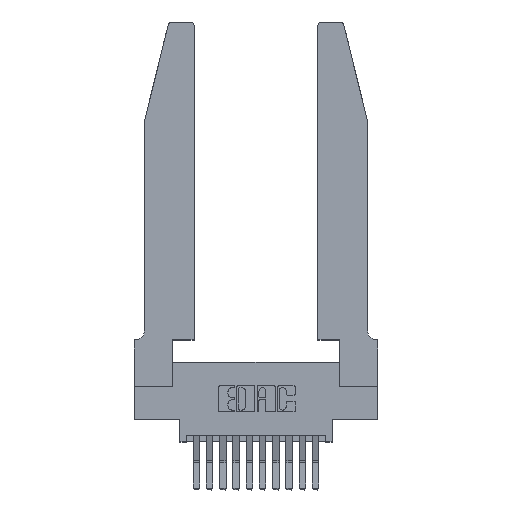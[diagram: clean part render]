
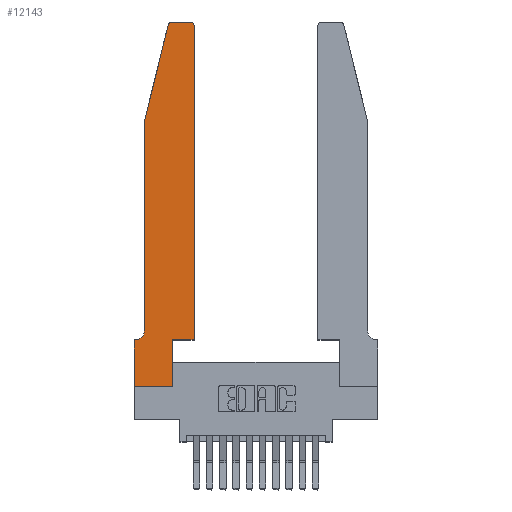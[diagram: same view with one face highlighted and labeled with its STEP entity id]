
A CAD part, top view. The second image highlights one B-rep face of the part: STEP entity #12143.
In plain terms, the highlighted planar face has unit normal (0, 0, 1).
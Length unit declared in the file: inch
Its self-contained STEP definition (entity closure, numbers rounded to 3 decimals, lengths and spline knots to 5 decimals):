
#3 = VERTEX_POINT ( 'NONE', #9684 ) ;
#420 = LINE ( 'NONE', #16414, #14131 ) ;
#710 = ORIENTED_EDGE ( 'NONE', *, *, #14507, .T. ) ;
#722 = DIRECTION ( 'NONE',  ( 1., 0., 0. ) ) ;
#805 = VERTEX_POINT ( 'NONE', #4292 ) ;
#1118 = DIRECTION ( 'NONE',  ( -1., 0., 0. ) ) ;
#1299 = EDGE_CURVE ( 'NONE', #12303, #10691, #420, .T. ) ;
#1308 = CARTESIAN_POINT ( 'NONE',  ( 0.4505, 0.35, 0.37 ) ) ;
#1601 = ORIENTED_EDGE ( 'NONE', *, *, #2215, .T. ) ;
#2215 = EDGE_CURVE ( 'NONE', #4727, #5094, #15937, .T. ) ;
#2238 = CARTESIAN_POINT ( 'NONE',  ( 0.0755, 2., 0.37 ) ) ;
#2670 = CARTESIAN_POINT ( 'NONE',  ( 0.0055, 0.35, 0.37 ) ) ;
#2739 = LINE ( 'NONE', #3442, #13275 ) ;
#3157 = LINE ( 'NONE', #16989, #16668 ) ;
#3193 = VERTEX_POINT ( 'NONE', #8471 ) ;
#3205 = ORIENTED_EDGE ( 'NONE', *, *, #13004, .T. ) ;
#3220 = CARTESIAN_POINT ( 'NONE',  ( 0.0755, 2., 0.37 ) ) ;
#3237 = LINE ( 'NONE', #15330, #13325 ) ;
#3442 = CARTESIAN_POINT ( 'NONE',  ( 0., 0., 0.37 ) ) ;
#3462 = ORIENTED_EDGE ( 'NONE', *, *, #9784, .T. ) ;
#3712 = ORIENTED_EDGE ( 'NONE', *, *, #1299, .T. ) ;
#3926 = CARTESIAN_POINT ( 'NONE',  ( 0., 0., 0.37 ) ) ;
#4292 = CARTESIAN_POINT ( 'NONE',  ( 0.2865, 0., 0.37 ) ) ;
#4449 = ORIENTED_EDGE ( 'NONE', *, *, #14977, .T. ) ;
#4578 = EDGE_LOOP ( 'NONE', ( #3462, #12439, #3205, #4449, #11653, #3712, #5578, #15171, #8110, #15825, #710, #1601 ) ) ;
#4727 = VERTEX_POINT ( 'NONE', #11401 ) ;
#4792 = DIRECTION ( 'NONE',  ( -0.239, -0.971, 0. ) ) ;
#5094 = VERTEX_POINT ( 'NONE', #14942 ) ;
#5296 = DIRECTION ( 'NONE',  ( 1., 0., 0. ) ) ;
#5457 = AXIS2_PLACEMENT_3D ( 'NONE', #6131, #8782, #722 ) ;
#5578 = ORIENTED_EDGE ( 'NONE', *, *, #13606, .T. ) ;
#5979 = AXIS2_PLACEMENT_3D ( 'NONE', #15383, #7617, #16695 ) ;
#6131 = CARTESIAN_POINT ( 'NONE',  ( 0., 0.35, 0.37 ) ) ;
#6413 = DIRECTION ( 'NONE',  ( 0., 1., 0. ) ) ;
#6873 = CARTESIAN_POINT ( 'NONE',  ( 0.0755, 2., 0.37 ) ) ;
#7020 = EDGE_CURVE ( 'NONE', #9657, #12303, #12777, .T. ) ;
#7208 = DIRECTION ( 'NONE',  ( 0., 0., -1. ) ) ;
#7261 = EDGE_CURVE ( 'NONE', #14782, #3, #12577, .T. ) ;
#7352 = PLANE ( 'NONE',  #5457 ) ;
#7617 = DIRECTION ( 'NONE',  ( 0., 0., 1. ) ) ;
#8110 = ORIENTED_EDGE ( 'NONE', *, *, #15458, .T. ) ;
#8471 = CARTESIAN_POINT ( 'NONE',  ( 0., 0., 0.37 ) ) ;
#8506 = VERTEX_POINT ( 'NONE', #6873 ) ;
#8766 = CARTESIAN_POINT ( 'NONE',  ( 0.284, 2.75, 0.37 ) ) ;
#8782 = DIRECTION ( 'NONE',  ( 0., 0., 1. ) ) ;
#9070 = VECTOR ( 'NONE', #5296, 39.37008 ) ;
#9521 = LINE ( 'NONE', #3220, #16013 ) ;
#9524 = VERTEX_POINT ( 'NONE', #16996 ) ;
#9657 = VERTEX_POINT ( 'NONE', #12226 ) ;
#9684 = CARTESIAN_POINT ( 'NONE',  ( 0.4505, 0.35, 0.37 ) ) ;
#9725 = LINE ( 'NONE', #12959, #13215 ) ;
#9784 = EDGE_CURVE ( 'NONE', #5094, #10909, #3237, .T. ) ;
#9810 = EDGE_CURVE ( 'NONE', #10909, #9524, #9826, .T. ) ;
#9826 = CIRCLE ( 'NONE', #5979, 0.03 ) ;
#10176 = DIRECTION ( 'NONE',  ( 0., -1., 0. ) ) ;
#10691 = VERTEX_POINT ( 'NONE', #16097 ) ;
#10765 = VECTOR ( 'NONE', #15686, 39.37008 ) ;
#10909 = VERTEX_POINT ( 'NONE', #8766 ) ;
#11065 = CARTESIAN_POINT ( 'NONE',  ( 0.2865, 0.35, 0.37 ) ) ;
#11401 = CARTESIAN_POINT ( 'NONE',  ( 0.4505, 2.72, 0.37 ) ) ;
#11653 = ORIENTED_EDGE ( 'NONE', *, *, #7020, .T. ) ;
#11818 = FACE_OUTER_BOUND ( 'NONE', #4578, .T. ) ;
#12143 = ADVANCED_FACE ( 'NONE', ( #11818 ), #7352, .T. ) ;
#12226 = CARTESIAN_POINT ( 'NONE',  ( 0.0755, 0.42, 0.37 ) ) ;
#12303 = VERTEX_POINT ( 'NONE', #2670 ) ;
#12439 = ORIENTED_EDGE ( 'NONE', *, *, #9810, .T. ) ;
#12577 = LINE ( 'NONE', #1308, #9070 ) ;
#12652 = DIRECTION ( 'NONE',  ( 0., -1., 0. ) ) ;
#12777 = CIRCLE ( 'NONE', #14153, 0.07 ) ;
#12823 = VECTOR ( 'NONE', #10176, 39.37008 ) ;
#12959 = CARTESIAN_POINT ( 'NONE',  ( 0.2865, 0.35, 0.37 ) ) ;
#12963 = DIRECTION ( 'NONE',  ( 0., 0., 1. ) ) ;
#13004 = EDGE_CURVE ( 'NONE', #9524, #8506, #9521, .T. ) ;
#13186 = DIRECTION ( 'NONE',  ( 0., 1., 0. ) ) ;
#13215 = VECTOR ( 'NONE', #6413, 39.37008 ) ;
#13230 = LINE ( 'NONE', #2238, #12823 ) ;
#13275 = VECTOR ( 'NONE', #12652, 39.37008 ) ;
#13325 = VECTOR ( 'NONE', #16648, 39.37008 ) ;
#13606 = EDGE_CURVE ( 'NONE', #10691, #3193, #2739, .T. ) ;
#14131 = VECTOR ( 'NONE', #1118, 39.37008 ) ;
#14153 = AXIS2_PLACEMENT_3D ( 'NONE', #14984, #7208, #16304 ) ;
#14212 = LINE ( 'NONE', #3926, #10765 ) ;
#14314 = AXIS2_PLACEMENT_3D ( 'NONE', #14321, #12963, #15377 ) ;
#14321 = CARTESIAN_POINT ( 'NONE',  ( 0.4205, 2.72, 0.37 ) ) ;
#14507 = EDGE_CURVE ( 'NONE', #3, #4727, #3157, .T. ) ;
#14782 = VERTEX_POINT ( 'NONE', #11065 ) ;
#14942 = CARTESIAN_POINT ( 'NONE',  ( 0.4205, 2.75, 0.37 ) ) ;
#14977 = EDGE_CURVE ( 'NONE', #8506, #9657, #13230, .T. ) ;
#14984 = CARTESIAN_POINT ( 'NONE',  ( 0.0055, 0.42, 0.37 ) ) ;
#15131 = EDGE_CURVE ( 'NONE', #3193, #805, #14212, .T. ) ;
#15171 = ORIENTED_EDGE ( 'NONE', *, *, #15131, .T. ) ;
#15330 = CARTESIAN_POINT ( 'NONE',  ( 0.2605, 2.75, 0.37 ) ) ;
#15377 = DIRECTION ( 'NONE',  ( 1., 0., 0. ) ) ;
#15383 = CARTESIAN_POINT ( 'NONE',  ( 0.284, 2.72, 0.37 ) ) ;
#15458 = EDGE_CURVE ( 'NONE', #805, #14782, #9725, .T. ) ;
#15686 = DIRECTION ( 'NONE',  ( 1., 0., 0. ) ) ;
#15825 = ORIENTED_EDGE ( 'NONE', *, *, #7261, .T. ) ;
#15937 = CIRCLE ( 'NONE', #14314, 0.03 ) ;
#16013 = VECTOR ( 'NONE', #4792, 39.37008 ) ;
#16097 = CARTESIAN_POINT ( 'NONE',  ( 0., 0.35, 0.37 ) ) ;
#16304 = DIRECTION ( 'NONE',  ( -1., 0., 0. ) ) ;
#16414 = CARTESIAN_POINT ( 'NONE',  ( 0.0755, 0.35, 0.37 ) ) ;
#16648 = DIRECTION ( 'NONE',  ( -1., 0., 0. ) ) ;
#16668 = VECTOR ( 'NONE', #13186, 39.37008 ) ;
#16695 = DIRECTION ( 'NONE',  ( 1., 0., 0. ) ) ;
#16989 = CARTESIAN_POINT ( 'NONE',  ( 0.4505, 0.35, 0.37 ) ) ;
#16996 = CARTESIAN_POINT ( 'NONE',  ( 0.25487, 2.72718, 0.37 ) ) ;
